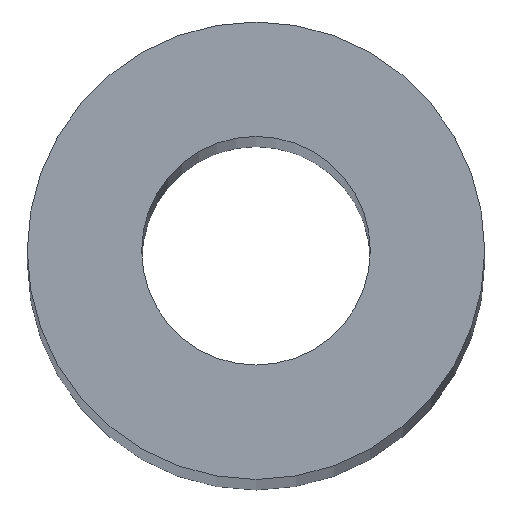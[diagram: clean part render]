
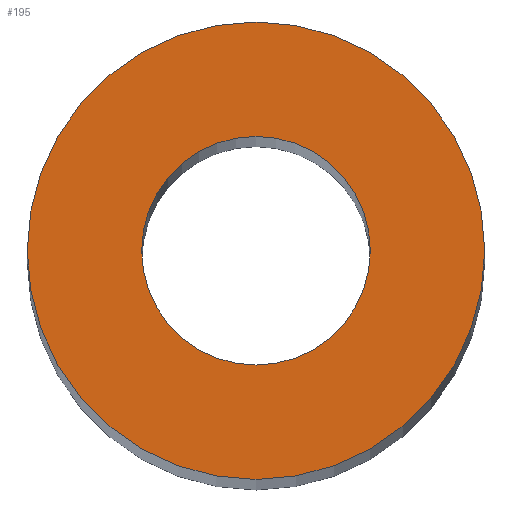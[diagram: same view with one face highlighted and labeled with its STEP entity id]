
A CAD part, top view. The second image highlights one B-rep face of the part: STEP entity #195.
In plain terms, the highlighted planar face has unit normal (0, 0, 1).
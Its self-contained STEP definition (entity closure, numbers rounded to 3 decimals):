
#16=FACE_BOUND('',#49,.T.);
#25=PLANE('',#224);
#36=FACE_OUTER_BOUND('',#48,.T.);
#48=EDGE_LOOP('',(#175));
#49=EDGE_LOOP('',(#176));
#93=CIRCLE('',#213,3.5);
#94=CIRCLE('',#222,7.);
#97=VERTEX_POINT('',#282);
#110=VERTEX_POINT('',#323);
#114=EDGE_CURVE('',#97,#97,#93,.T.);
#133=EDGE_CURVE('',#110,#110,#94,.F.);
#175=ORIENTED_EDGE('',*,*,#133,.T.);
#176=ORIENTED_EDGE('',*,*,#114,.T.);
#195=ADVANCED_FACE('',(#36,#16),#25,.T.);
#213=AXIS2_PLACEMENT_3D('',#284,#233,#234);
#222=AXIS2_PLACEMENT_3D('',#324,#269,#270);
#224=AXIS2_PLACEMENT_3D('',#328,#274,#275);
#233=DIRECTION('center_axis',(0.,0.,-1.));
#234=DIRECTION('ref_axis',(1.,0.,0.));
#269=DIRECTION('center_axis',(0.,0.,-1.));
#270=DIRECTION('ref_axis',(1.,0.,0.));
#274=DIRECTION('center_axis',(0.,0.,1.));
#275=DIRECTION('ref_axis',(1.,0.,0.));
#282=CARTESIAN_POINT('',(36.5,25.,185.));
#284=CARTESIAN_POINT('Origin',(40.,25.,185.));
#323=CARTESIAN_POINT('',(33.,25.,185.));
#324=CARTESIAN_POINT('Origin',(40.,25.,185.));
#328=CARTESIAN_POINT('Origin',(40.,25.,185.));
